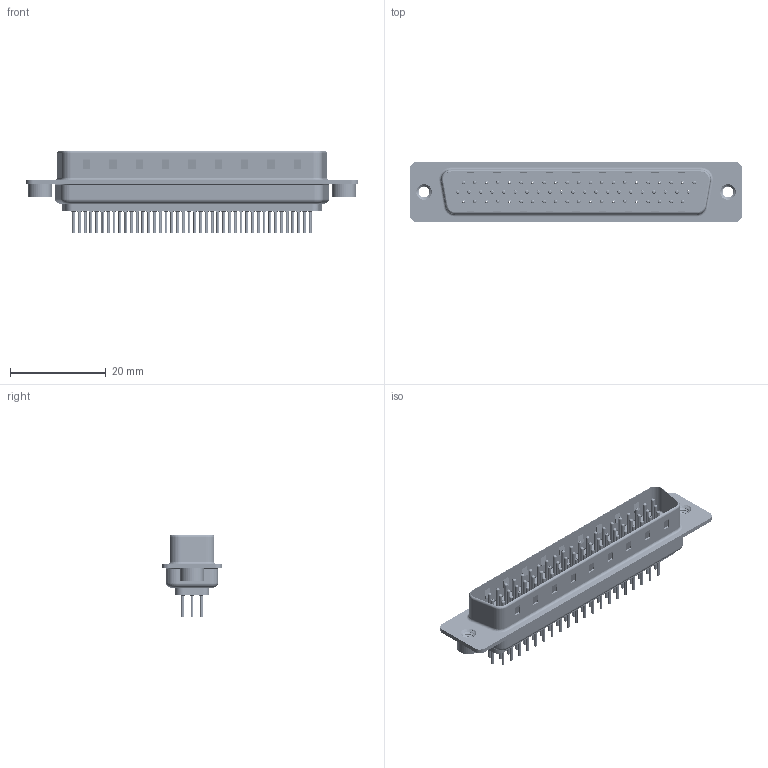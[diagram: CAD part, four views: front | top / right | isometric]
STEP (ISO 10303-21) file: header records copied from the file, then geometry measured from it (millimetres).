
FILE_DESCRIPTION (( 'STEP AP203' ), '1' );
FILE_NAME ('637-062-230-242.STEP', '2020-07-18T03:29:28', ( '' ), ( '' ), 'SwSTEP 2.0', 'SolidWorks 2020', '' );
FILE_SCHEMA (( 'CONFIG_CONTROL_DESIGN' ));
Length unit declared in the file: millimetre
Products named in the file (8): 637 Contact Row 2_30; 637 Shell Front_62 Contacts; 637-062-230-242; 637 Contact Row 3_30; 637 Shell Rear_62 Contacts; 637 Housing_62 Contacts; 637 4-40 Threaded Rivet; 637 Contact Row 1_30
Assembly tree (67 placements, depth 2):
  637-062-230-242
    637 Housing_62 Contacts
    637 Shell Front_62 Contacts
    637 Shell Rear_62 Contacts
    637 Contact Row 1_30  x21
    637 Contact Row 2_30  x21
    637 Contact Row 3_30  x20
    637 4-40 Threaded Rivet  x2
Bounding box: 69.4 x 12.6 x 17.25 mm (x, y, z)
Volume: 3689.2 mm3; surface area: 13622.8 mm2
Topology: 67 solids, 67 shells, 6612 faces, 17487 edges, 10772 vertices
Faces by surface type: cylinder 2435, torus 1848, plane 1691, cone 632, bspline 6
Entity records: 39312 total; most frequent: CARTESIAN_POINT 8179, DIRECTION 6509, ORIENTED_EDGE 5618, EDGE_CURVE 2809, AXIS2_PLACEMENT_3D 2631, VERTEX_POINT 1805, EDGE_LOOP 1458, CIRCLE 1413
